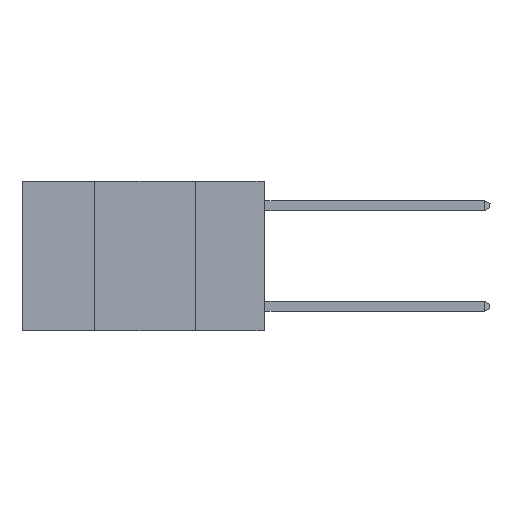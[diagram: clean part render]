
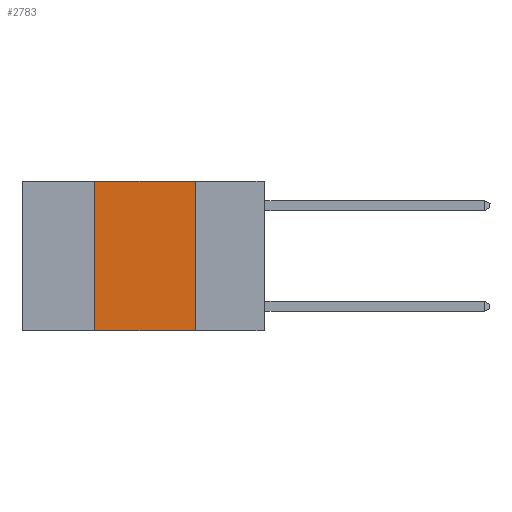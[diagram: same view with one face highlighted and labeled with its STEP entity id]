
A CAD part, left-side view. The second image highlights one B-rep face of the part: STEP entity #2783.
In plain terms, the highlighted planar face has unit normal (-1, 0, 0).
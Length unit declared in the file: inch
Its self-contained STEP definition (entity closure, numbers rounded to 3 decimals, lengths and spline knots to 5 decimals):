
#123 = DIRECTION ( 'NONE',  ( 0., -1., 0. ) ) ;
#305 = ORIENTED_EDGE ( 'NONE', *, *, #2416, .F. ) ;
#419 = VERTEX_POINT ( 'NONE', #5057 ) ;
#663 = LINE ( 'NONE', #3142, #2400 ) ;
#1150 = CARTESIAN_POINT ( 'NONE',  ( 0., 0.6, 0. ) ) ;
#1756 = CARTESIAN_POINT ( 'NONE',  ( 0., 0.17, -0.37 ) ) ;
#2363 = EDGE_CURVE ( 'NONE', #5933, #5693, #4370, .T. ) ;
#2400 = VECTOR ( 'NONE', #8149, 39.37008 ) ;
#2416 = EDGE_CURVE ( 'NONE', #419, #3187, #6417, .T. ) ;
#2783 = ADVANCED_FACE ( 'NONE', ( #3858 ), #10313, .F. ) ;
#3100 = DIRECTION ( 'NONE',  ( 1., 0., 0. ) ) ;
#3142 = CARTESIAN_POINT ( 'NONE',  ( 0., 0.6, -0.37 ) ) ;
#3187 = VERTEX_POINT ( 'NONE', #1756 ) ;
#3191 = VECTOR ( 'NONE', #123, 39.37008 ) ;
#3456 = EDGE_CURVE ( 'NONE', #5933, #3187, #663, .T. ) ;
#3858 = FACE_OUTER_BOUND ( 'NONE', #10087, .T. ) ;
#3909 = CARTESIAN_POINT ( 'NONE',  ( 0., 0.6, 0. ) ) ;
#4370 = LINE ( 'NONE', #7587, #7456 ) ;
#4680 = DIRECTION ( 'NONE',  ( 0., 0., -1. ) ) ;
#4845 = EDGE_CURVE ( 'NONE', #5693, #419, #4940, .T. ) ;
#4940 = LINE ( 'NONE', #1150, #3191 ) ;
#5057 = CARTESIAN_POINT ( 'NONE',  ( 0., 0.17, 0. ) ) ;
#5613 = DIRECTION ( 'NONE',  ( 0., 0., -1. ) ) ;
#5693 = VERTEX_POINT ( 'NONE', #10037 ) ;
#5933 = VERTEX_POINT ( 'NONE', #9448 ) ;
#6417 = LINE ( 'NONE', #8711, #9853 ) ;
#6866 = ORIENTED_EDGE ( 'NONE', *, *, #3456, .T. ) ;
#7253 = AXIS2_PLACEMENT_3D ( 'NONE', #3909, #3100, #4680 ) ;
#7456 = VECTOR ( 'NONE', #7695, 39.37008 ) ;
#7587 = CARTESIAN_POINT ( 'NONE',  ( 0., 0.42, 0. ) ) ;
#7695 = DIRECTION ( 'NONE',  ( 0., 0., 1. ) ) ;
#8149 = DIRECTION ( 'NONE',  ( 0., -1., 0. ) ) ;
#8711 = CARTESIAN_POINT ( 'NONE',  ( 0., 0.17, 0. ) ) ;
#9034 = ORIENTED_EDGE ( 'NONE', *, *, #2363, .F. ) ;
#9448 = CARTESIAN_POINT ( 'NONE',  ( 0., 0.42, -0.37 ) ) ;
#9473 = ORIENTED_EDGE ( 'NONE', *, *, #4845, .F. ) ;
#9853 = VECTOR ( 'NONE', #5613, 39.37008 ) ;
#10037 = CARTESIAN_POINT ( 'NONE',  ( 0., 0.42, 0. ) ) ;
#10087 = EDGE_LOOP ( 'NONE', ( #305, #9473, #9034, #6866 ) ) ;
#10313 = PLANE ( 'NONE',  #7253 ) ;
